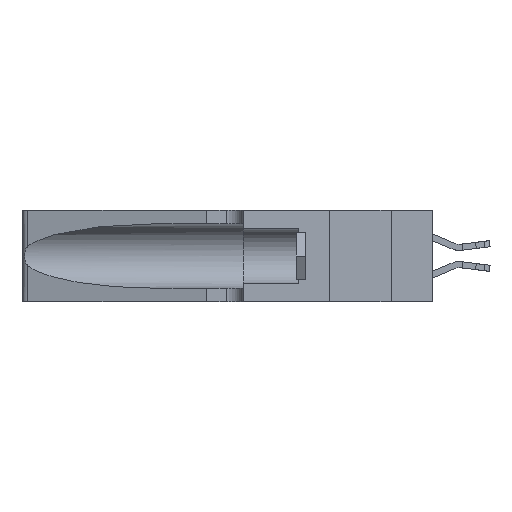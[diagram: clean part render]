
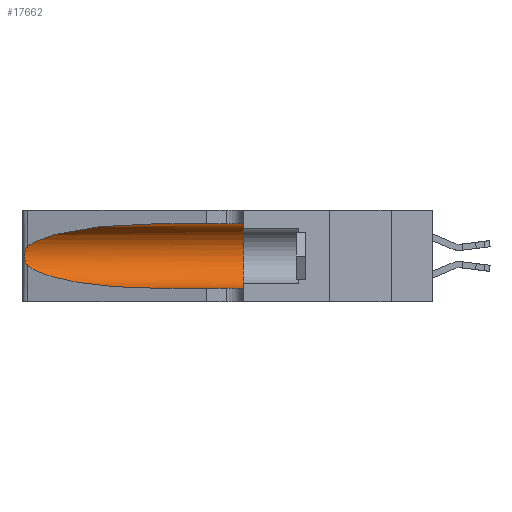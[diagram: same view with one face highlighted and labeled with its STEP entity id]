
A CAD part, left-side view. The second image highlights one B-rep face of the part: STEP entity #17662.
In plain terms, the highlighted cylindrical face has radius 3.308 mm (diameter 6.617 mm), a partial arc.
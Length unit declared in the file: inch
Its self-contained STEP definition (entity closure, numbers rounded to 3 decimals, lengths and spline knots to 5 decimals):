
#133 = CARTESIAN_POINT ( 'NONE',  ( 0.1305, 1.61858, 0.05475 ) ) ;
#157 = FACE_OUTER_BOUND ( 'NONE', #6514, .T. ) ;
#203 = CARTESIAN_POINT ( 'NONE',  ( 0.25487, 1.22718, 0.22369 ) ) ;
#289 = ORIENTED_EDGE ( 'NONE', *, *, #25613, .T. ) ;
#697 = CARTESIAN_POINT ( 'NONE',  ( 0.1305, 1.61858, 0.31525 ) ) ;
#704 = VERTEX_POINT ( 'NONE', #2116 ) ;
#1386 = DIRECTION ( 'NONE',  ( 0., 1., 0. ) ) ;
#1459 = ORIENTED_EDGE ( 'NONE', *, *, #2922, .T. ) ;
#1865 = CARTESIAN_POINT ( 'NONE',  ( 0.26017, 1.23833, 0.17102 ) ) ;
#2116 = CARTESIAN_POINT ( 'NONE',  ( 0.1305, 0.35, 0.31525 ) ) ;
#2243 = ORIENTED_EDGE ( 'NONE', *, *, #12969, .F. ) ;
#2328 = VERTEX_POINT ( 'NONE', #21218 ) ;
#2420 = DIRECTION ( 'NONE',  ( 0., -1., 0. ) ) ;
#2922 = EDGE_CURVE ( 'NONE', #3111, #7912, #14141, .T. ) ;
#3053 = EDGE_CURVE ( 'NONE', #704, #2328, #5504, .T. ) ;
#3111 = VERTEX_POINT ( 'NONE', #6093 ) ;
#3497 = ORIENTED_EDGE ( 'NONE', *, *, #16332, .T. ) ;
#3608 =( BOUNDED_CURVE ( )  B_SPLINE_CURVE ( 3, ( #4601, #27115, #11526, #203 ),
 .UNSPECIFIED., .F., .F. ) 
 B_SPLINE_CURVE_WITH_KNOTS ( ( 4, 4 ),
 ( 1.5708, 2.84003 ),
 .UNSPECIFIED. ) 
 CURVE ( )  GEOMETRIC_REPRESENTATION_ITEM ( )  RATIONAL_B_SPLINE_CURVE ( ( 1., 0.87, 0.87, 1. ) ) 
 REPRESENTATION_ITEM ( '' )  );
#4071 = CARTESIAN_POINT ( 'NONE',  ( 0.25555, 1.22994, 0.2215 ) ) ;
#4172 = CARTESIAN_POINT ( 'NONE',  ( 0.25789, 1.23486, 0.15765 ) ) ;
#4524 = AXIS2_PLACEMENT_3D ( 'NONE', #5120, #23044, #9664 ) ;
#4601 = CARTESIAN_POINT ( 'NONE',  ( 0.1305, 0.72297, 0.31525 ) ) ;
#5120 = CARTESIAN_POINT ( 'NONE',  ( 0.1305, 1.61858, 0.185 ) ) ;
#5504 = CIRCLE ( 'NONE', #22210, 0.13025 ) ;
#5516 = CARTESIAN_POINT ( 'NONE',  ( 0.18966, 0.96281, 0.05475 ) ) ;
#5897 = ORIENTED_EDGE ( 'NONE', *, *, #7262, .T. ) ;
#6093 = CARTESIAN_POINT ( 'NONE',  ( 0.25487, 1.22718, 0.14631 ) ) ;
#6452 = CARTESIAN_POINT ( 'NONE',  ( 0.25555, 1.22993, 0.14849 ) ) ;
#6514 = EDGE_LOOP ( 'NONE', ( #5897, #289, #1459, #3497, #6751, #2243 ) ) ;
#6751 = ORIENTED_EDGE ( 'NONE', *, *, #3053, .F. ) ;
#7262 = EDGE_CURVE ( 'NONE', #13905, #23493, #3608, .T. ) ;
#7912 = VERTEX_POINT ( 'NONE', #15923 ) ;
#9664 = DIRECTION ( 'NONE',  ( 0., 0., -1. ) ) ;
#10061 = CARTESIAN_POINT ( 'NONE',  ( 0.25487, 1.22718, 0.14631 ) ) ;
#10403 = VECTOR ( 'NONE', #23218, 39.37008 ) ;
#10907 = CARTESIAN_POINT ( 'NONE',  ( 0.25787, 1.23484, 0.2124 ) ) ;
#11526 = CARTESIAN_POINT ( 'NONE',  ( 0.2373, 1.15595, 0.28018 ) ) ;
#11956 = CARTESIAN_POINT ( 'NONE',  ( 0.1305, 0.72297, 0.31525 ) ) ;
#12969 = EDGE_CURVE ( 'NONE', #13905, #704, #17065, .T. ) ;
#13060 = CARTESIAN_POINT ( 'NONE',  ( 0.25487, 1.22718, 0.22369 ) ) ;
#13156 = CARTESIAN_POINT ( 'NONE',  ( 0.26018, 1.23835, 0.19895 ) ) ;
#13905 = VERTEX_POINT ( 'NONE', #11956 ) ;
#14141 =( BOUNDED_CURVE ( )  B_SPLINE_CURVE ( 3, ( #10061, #23431, #5516, #25673 ),
 .UNSPECIFIED., .F., .T. ) 
 B_SPLINE_CURVE_WITH_KNOTS ( ( 4, 4 ),
 ( 3.44316, 4.71239 ),
 .UNSPECIFIED. ) 
 CURVE ( )  GEOMETRIC_REPRESENTATION_ITEM ( )  RATIONAL_B_SPLINE_CURVE ( ( 1., 0.87, 0.87, 1. ) ) 
 REPRESENTATION_ITEM ( '' )  );
#14955 = CARTESIAN_POINT ( 'NONE',  ( 0.1305, 0.35, 0.185 ) ) ;
#15416 = CARTESIAN_POINT ( 'NONE',  ( 0.26075, 1.23896, 0.178 ) ) ;
#15923 = CARTESIAN_POINT ( 'NONE',  ( 0.1305, 0.72297, 0.05475 ) ) ;
#16332 = EDGE_CURVE ( 'NONE', #7912, #2328, #17213, .T. ) ;
#17065 = LINE ( 'NONE', #697, #10403 ) ;
#17213 = LINE ( 'NONE', #133, #27640 ) ;
#17217 = DIRECTION ( 'NONE',  ( 0., 0., 1. ) ) ;
#17662 = ADVANCED_FACE ( 'NONE', ( #157 ), #28600, .F. ) ;
#17668 = CARTESIAN_POINT ( 'NONE',  ( 0.25856, 1.23593, 0.16098 ) ) ;
#19904 = CARTESIAN_POINT ( 'NONE',  ( 0.25639, 1.23186, 0.15144 ) ) ;
#21218 = CARTESIAN_POINT ( 'NONE',  ( 0.1305, 0.35, 0.05475 ) ) ;
#22114 = CARTESIAN_POINT ( 'NONE',  ( 0.25487, 1.22718, 0.14631 ) ) ;
#22210 = AXIS2_PLACEMENT_3D ( 'NONE', #14955, #1386, #17217 ) ;
#22400 = CARTESIAN_POINT ( 'NONE',  ( 0.25487, 1.22718, 0.22369 ) ) ;
#23044 = DIRECTION ( 'NONE',  ( 0., -1., 0. ) ) ;
#23218 = DIRECTION ( 'NONE',  ( 0., -1., 0. ) ) ;
#23222 = B_SPLINE_CURVE_WITH_KNOTS ( 'NONE', 3,
 ( #13060, #4071, #24275, #10907, #26508, #13156, #28753, #15416, #1865, #17668, #4172, #19904, #6452, #22114 ),
 .UNSPECIFIED., .F., .F.,
 ( 4, 2, 2, 2, 2, 2, 4 ),
 ( 0., 0.00027, 0.00053, 0.00107, 0.0016, 0.00187, 0.00214 ),
 .UNSPECIFIED. ) ;
#23431 = CARTESIAN_POINT ( 'NONE',  ( 0.2373, 1.15595, 0.08982 ) ) ;
#23493 = VERTEX_POINT ( 'NONE', #22400 ) ;
#24275 = CARTESIAN_POINT ( 'NONE',  ( 0.25639, 1.23184, 0.21858 ) ) ;
#25613 = EDGE_CURVE ( 'NONE', #23493, #3111, #23222, .T. ) ;
#25673 = CARTESIAN_POINT ( 'NONE',  ( 0.1305, 0.72297, 0.05475 ) ) ;
#26508 = CARTESIAN_POINT ( 'NONE',  ( 0.25854, 1.2359, 0.20912 ) ) ;
#27115 = CARTESIAN_POINT ( 'NONE',  ( 0.18966, 0.96281, 0.31525 ) ) ;
#27640 = VECTOR ( 'NONE', #2420, 39.37008 ) ;
#28600 = CYLINDRICAL_SURFACE ( 'NONE', #4524, 0.13025 ) ;
#28753 = CARTESIAN_POINT ( 'NONE',  ( 0.26075, 1.23896, 0.19203 ) ) ;
